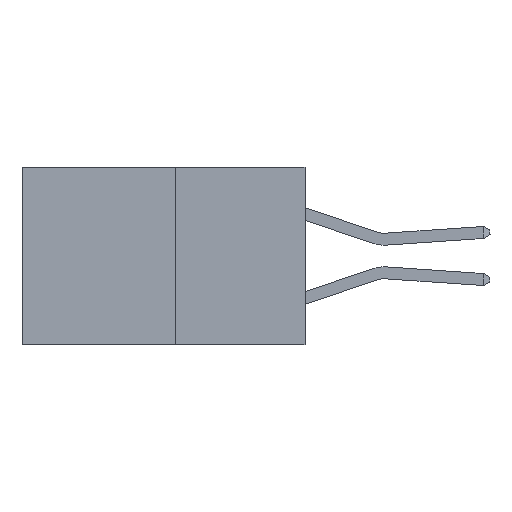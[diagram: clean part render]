
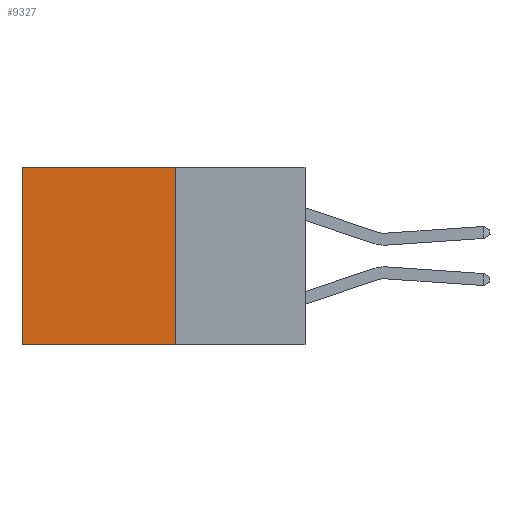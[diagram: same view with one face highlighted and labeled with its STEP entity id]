
A CAD part, left-side view. The second image highlights one B-rep face of the part: STEP entity #9327.
In plain terms, the highlighted planar face has unit normal (-1, 0, 0).
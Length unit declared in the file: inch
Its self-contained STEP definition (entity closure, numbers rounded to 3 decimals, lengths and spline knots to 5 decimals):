
#1157 = CARTESIAN_POINT ( 'NONE',  ( 0.277, 0.27, -0.37 ) ) ;
#1335 = ORIENTED_EDGE ( 'NONE', *, *, #3697, .F. ) ;
#1579 = LINE ( 'NONE', #10296, #16293 ) ;
#2373 = DIRECTION ( 'NONE',  ( 1., 0., 0. ) ) ;
#3397 = VERTEX_POINT ( 'NONE', #15299 ) ;
#3697 = EDGE_CURVE ( 'NONE', #9889, #14814, #1579, .T. ) ;
#3729 = ORIENTED_EDGE ( 'NONE', *, *, #11244, .T. ) ;
#4308 = CARTESIAN_POINT ( 'NONE',  ( 0.277, 0.59, -0.37 ) ) ;
#4791 = CARTESIAN_POINT ( 'NONE',  ( 0.277, 0.27, 0. ) ) ;
#7044 = EDGE_LOOP ( 'NONE', ( #18086, #1335, #10125, #3729 ) ) ;
#7203 = VERTEX_POINT ( 'NONE', #4791 ) ;
#7844 = LINE ( 'NONE', #11230, #14932 ) ;
#8315 = EDGE_CURVE ( 'NONE', #3397, #14814, #16571, .T. ) ;
#8478 = DIRECTION ( 'NONE',  ( 0., 0., -1. ) ) ;
#8617 = VECTOR ( 'NONE', #15677, 39.37008 ) ;
#9327 = ADVANCED_FACE ( 'NONE', ( #10609 ), #9544, .F. ) ;
#9480 = CARTESIAN_POINT ( 'NONE',  ( 0.277, 0.27, -0.37 ) ) ;
#9544 = PLANE ( 'NONE',  #17167 ) ;
#9889 = VERTEX_POINT ( 'NONE', #1157 ) ;
#10125 = ORIENTED_EDGE ( 'NONE', *, *, #11300, .F. ) ;
#10296 = CARTESIAN_POINT ( 'NONE',  ( 0.277, 0.27, -0.37 ) ) ;
#10609 = FACE_OUTER_BOUND ( 'NONE', #7044, .T. ) ;
#11230 = CARTESIAN_POINT ( 'NONE',  ( 0.277, 0.27, 0. ) ) ;
#11244 = EDGE_CURVE ( 'NONE', #7203, #3397, #7844, .T. ) ;
#11300 = EDGE_CURVE ( 'NONE', #7203, #9889, #14485, .T. ) ;
#12413 = DIRECTION ( 'NONE',  ( 0., 0., -1. ) ) ;
#12664 = DIRECTION ( 'NONE',  ( 0., 1., 0. ) ) ;
#14053 = VECTOR ( 'NONE', #8478, 39.37008 ) ;
#14485 = LINE ( 'NONE', #15537, #14053 ) ;
#14814 = VERTEX_POINT ( 'NONE', #15232 ) ;
#14932 = VECTOR ( 'NONE', #12664, 39.37008 ) ;
#15232 = CARTESIAN_POINT ( 'NONE',  ( 0.277, 0.59, -0.37 ) ) ;
#15299 = CARTESIAN_POINT ( 'NONE',  ( 0.277, 0.59, 0. ) ) ;
#15537 = CARTESIAN_POINT ( 'NONE',  ( 0.277, 0.27, -0.37 ) ) ;
#15677 = DIRECTION ( 'NONE',  ( 0., 0., -1. ) ) ;
#16293 = VECTOR ( 'NONE', #17227, 39.37008 ) ;
#16571 = LINE ( 'NONE', #4308, #8617 ) ;
#17167 = AXIS2_PLACEMENT_3D ( 'NONE', #9480, #2373, #12413 ) ;
#17227 = DIRECTION ( 'NONE',  ( 0., 1., 0. ) ) ;
#18086 = ORIENTED_EDGE ( 'NONE', *, *, #8315, .T. ) ;
